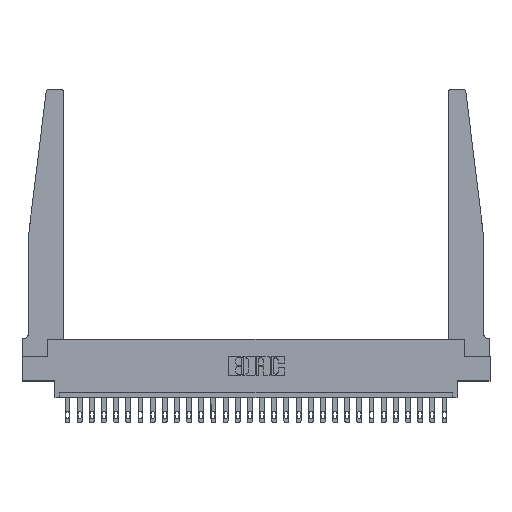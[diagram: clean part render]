
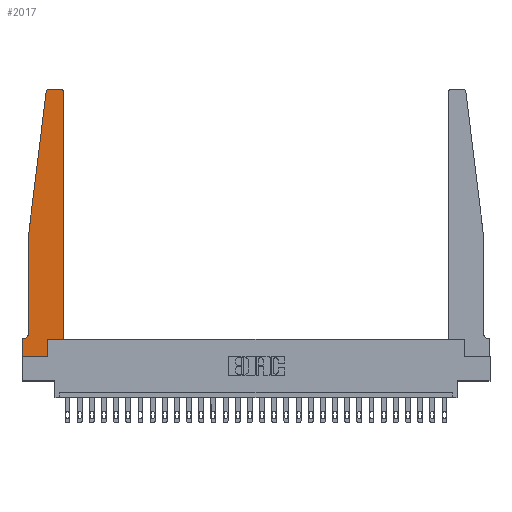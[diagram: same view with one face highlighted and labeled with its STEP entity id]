
A CAD part, top view. The second image highlights one B-rep face of the part: STEP entity #2017.
In plain terms, the highlighted planar face has unit normal (0, 0, 1).
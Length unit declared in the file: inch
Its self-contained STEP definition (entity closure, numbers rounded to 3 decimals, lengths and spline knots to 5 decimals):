
#153 = VERTEX_POINT ( 'NONE', #6926 ) ;
#688 = EDGE_CURVE ( 'NONE', #153, #20181, #6774, .T. ) ;
#949 = DIRECTION ( 'NONE',  ( 1., 0., 0. ) ) ;
#1023 = DIRECTION ( 'NONE',  ( 1., 0., 0. ) ) ;
#1276 = DIRECTION ( 'NONE',  ( 1., 0., 0. ) ) ;
#1499 = VECTOR ( 'NONE', #18911, 39.37008 ) ;
#1725 = VECTOR ( 'NONE', #9892, 39.37008 ) ;
#1902 = VECTOR ( 'NONE', #8652, 39.37008 ) ;
#1983 = DIRECTION ( 'NONE',  ( 1., 0., 0. ) ) ;
#2017 = ADVANCED_FACE ( 'NONE', ( #8133 ), #22481, .T. ) ;
#2351 = VERTEX_POINT ( 'NONE', #23798 ) ;
#2578 = VECTOR ( 'NONE', #12641, 39.37008 ) ;
#2781 = VERTEX_POINT ( 'NONE', #5404 ) ;
#2815 = ORIENTED_EDGE ( 'NONE', *, *, #5220, .T. ) ;
#3028 = VECTOR ( 'NONE', #14323, 39.37008 ) ;
#3464 = CIRCLE ( 'NONE', #17606, 0.03 ) ;
#3658 = CARTESIAN_POINT ( 'NONE',  ( 0.395, 2.75, 0.37 ) ) ;
#4123 = DIRECTION ( 'NONE',  ( 0., 0., 1. ) ) ;
#4256 = VERTEX_POINT ( 'NONE', #21614 ) ;
#4697 = ORIENTED_EDGE ( 'NONE', *, *, #6695, .T. ) ;
#4855 = CARTESIAN_POINT ( 'NONE',  ( 0.065, 1.25, 0.37 ) ) ;
#4904 = CIRCLE ( 'NONE', #23738, 0.03 ) ;
#4925 = DIRECTION ( 'NONE',  ( -1., 0., 0. ) ) ;
#5220 = EDGE_CURVE ( 'NONE', #24139, #153, #24096, .T. ) ;
#5404 = CARTESIAN_POINT ( 'NONE',  ( 0.24675, 2.72367, 0.37 ) ) ;
#5732 = CARTESIAN_POINT ( 'NONE',  ( 0.065, 1.25, 0.37 ) ) ;
#6248 = VECTOR ( 'NONE', #4925, 39.37008 ) ;
#6348 = CARTESIAN_POINT ( 'NONE',  ( 0.065, 1.25, 0.37 ) ) ;
#6378 = CARTESIAN_POINT ( 'NONE',  ( 0.015, 0.1875, 0.37 ) ) ;
#6695 = EDGE_CURVE ( 'NONE', #21869, #18672, #23389, .T. ) ;
#6774 = CIRCLE ( 'NONE', #21768, 0.05 ) ;
#6926 = CARTESIAN_POINT ( 'NONE',  ( 0.065, 0.2375, 0.37 ) ) ;
#7299 = CARTESIAN_POINT ( 'NONE',  ( 0., 0., 0.37 ) ) ;
#7384 = LINE ( 'NONE', #11544, #8232 ) ;
#7668 = CARTESIAN_POINT ( 'NONE',  ( 0., 0.1875, 0.37 ) ) ;
#8133 = FACE_OUTER_BOUND ( 'NONE', #12264, .T. ) ;
#8232 = VECTOR ( 'NONE', #19854, 39.37008 ) ;
#8279 = ORIENTED_EDGE ( 'NONE', *, *, #19443, .T. ) ;
#8289 = CARTESIAN_POINT ( 'NONE',  ( 0.425, 0.18, 0.37 ) ) ;
#8652 = DIRECTION ( 'NONE',  ( -1., 0., 0. ) ) ;
#9482 = CARTESIAN_POINT ( 'NONE',  ( 0.425, 0.18, 0.37 ) ) ;
#9531 = EDGE_CURVE ( 'NONE', #9549, #21869, #7384, .T. ) ;
#9549 = VERTEX_POINT ( 'NONE', #26127 ) ;
#9683 = ORIENTED_EDGE ( 'NONE', *, *, #22347, .T. ) ;
#9767 = CARTESIAN_POINT ( 'NONE',  ( 0.015, 0.2375, 0.37 ) ) ;
#9844 = ORIENTED_EDGE ( 'NONE', *, *, #15108, .T. ) ;
#9892 = DIRECTION ( 'NONE',  ( 0., -1., 0. ) ) ;
#10423 = CARTESIAN_POINT ( 'NONE',  ( 0., 0.1875, 0.37 ) ) ;
#10529 = ORIENTED_EDGE ( 'NONE', *, *, #9531, .T. ) ;
#10806 = LINE ( 'NONE', #17089, #1902 ) ;
#11544 = CARTESIAN_POINT ( 'NONE',  ( 0.2605, 0.18, 0.37 ) ) ;
#11653 = DIRECTION ( 'NONE',  ( -1., 0., 0. ) ) ;
#12041 = ORIENTED_EDGE ( 'NONE', *, *, #12421, .T. ) ;
#12264 = EDGE_LOOP ( 'NONE', ( #24611, #25885, #12041, #2815, #14383, #9683, #8279, #25136, #10529, #4697, #9844, #26449 ) ) ;
#12421 = EDGE_CURVE ( 'NONE', #2781, #24139, #16924, .T. ) ;
#12641 = DIRECTION ( 'NONE',  ( -0.122, -0.992, 0. ) ) ;
#12710 = DIRECTION ( 'NONE',  ( 0., 0., 1. ) ) ;
#13148 = CARTESIAN_POINT ( 'NONE',  ( 0., 0., 0.37 ) ) ;
#13783 = DIRECTION ( 'NONE',  ( 0., 0., -1. ) ) ;
#14323 = DIRECTION ( 'NONE',  ( 0., 1., 0. ) ) ;
#14383 = ORIENTED_EDGE ( 'NONE', *, *, #688, .T. ) ;
#15018 = LINE ( 'NONE', #13148, #1499 ) ;
#15108 = EDGE_CURVE ( 'NONE', #18672, #4256, #22229, .T. ) ;
#15259 = EDGE_CURVE ( 'NONE', #4256, #25385, #3464, .T. ) ;
#16924 = LINE ( 'NONE', #4855, #2578 ) ;
#17089 = CARTESIAN_POINT ( 'NONE',  ( 0.25, 2.75, 0.37 ) ) ;
#17153 = VERTEX_POINT ( 'NONE', #19692 ) ;
#17498 = LINE ( 'NONE', #7299, #25557 ) ;
#17528 = AXIS2_PLACEMENT_3D ( 'NONE', #10423, #4123, #1983 ) ;
#17606 = AXIS2_PLACEMENT_3D ( 'NONE', #24236, #12710, #22887 ) ;
#17640 = CARTESIAN_POINT ( 'NONE',  ( 0.425, 0.18, 0.37 ) ) ;
#18672 = VERTEX_POINT ( 'NONE', #9482 ) ;
#18770 = CARTESIAN_POINT ( 'NONE',  ( 0.2605, 0.18, 0.37 ) ) ;
#18911 = DIRECTION ( 'NONE',  ( 0., -1., 0. ) ) ;
#18932 = EDGE_CURVE ( 'NONE', #25385, #2351, #10806, .T. ) ;
#19300 = DIRECTION ( 'NONE',  ( 0., 0., 1. ) ) ;
#19336 = VECTOR ( 'NONE', #1023, 39.37008 ) ;
#19443 = EDGE_CURVE ( 'NONE', #23202, #17153, #15018, .T. ) ;
#19469 = EDGE_CURVE ( 'NONE', #2351, #2781, #4904, .T. ) ;
#19692 = CARTESIAN_POINT ( 'NONE',  ( 0., 0., 0.37 ) ) ;
#19854 = DIRECTION ( 'NONE',  ( 0., 1., 0. ) ) ;
#20181 = VERTEX_POINT ( 'NONE', #6378 ) ;
#21154 = LINE ( 'NONE', #21279, #6248 ) ;
#21279 = CARTESIAN_POINT ( 'NONE',  ( 0.065, 0.1875, 0.37 ) ) ;
#21614 = CARTESIAN_POINT ( 'NONE',  ( 0.425, 2.72, 0.37 ) ) ;
#21768 = AXIS2_PLACEMENT_3D ( 'NONE', #9767, #13783, #11653 ) ;
#21869 = VERTEX_POINT ( 'NONE', #18770 ) ;
#22229 = LINE ( 'NONE', #8289, #3028 ) ;
#22347 = EDGE_CURVE ( 'NONE', #20181, #23202, #21154, .T. ) ;
#22481 = PLANE ( 'NONE',  #17528 ) ;
#22887 = DIRECTION ( 'NONE',  ( 1., 0., 0. ) ) ;
#23050 = CARTESIAN_POINT ( 'NONE',  ( 0.27653, 2.72, 0.37 ) ) ;
#23202 = VERTEX_POINT ( 'NONE', #7668 ) ;
#23389 = LINE ( 'NONE', #17640, #19336 ) ;
#23738 = AXIS2_PLACEMENT_3D ( 'NONE', #23050, #19300, #949 ) ;
#23798 = CARTESIAN_POINT ( 'NONE',  ( 0.27653, 2.75, 0.37 ) ) ;
#24063 = EDGE_CURVE ( 'NONE', #17153, #9549, #17498, .T. ) ;
#24096 = LINE ( 'NONE', #5732, #1725 ) ;
#24139 = VERTEX_POINT ( 'NONE', #6348 ) ;
#24236 = CARTESIAN_POINT ( 'NONE',  ( 0.395, 2.72, 0.37 ) ) ;
#24611 = ORIENTED_EDGE ( 'NONE', *, *, #18932, .T. ) ;
#25136 = ORIENTED_EDGE ( 'NONE', *, *, #24063, .T. ) ;
#25385 = VERTEX_POINT ( 'NONE', #3658 ) ;
#25557 = VECTOR ( 'NONE', #1276, 39.37008 ) ;
#25885 = ORIENTED_EDGE ( 'NONE', *, *, #19469, .T. ) ;
#26127 = CARTESIAN_POINT ( 'NONE',  ( 0.2605, 0., 0.37 ) ) ;
#26449 = ORIENTED_EDGE ( 'NONE', *, *, #15259, .T. ) ;
